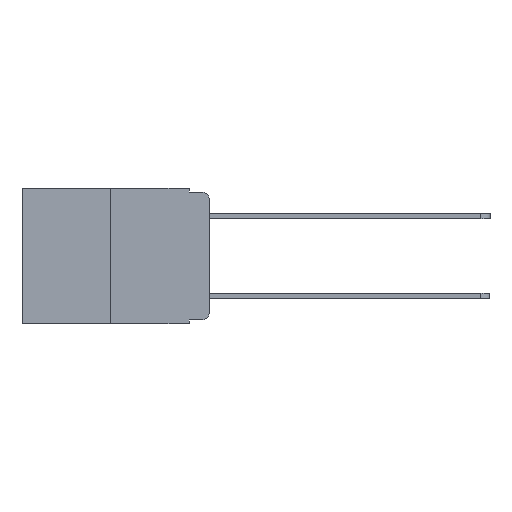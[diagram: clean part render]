
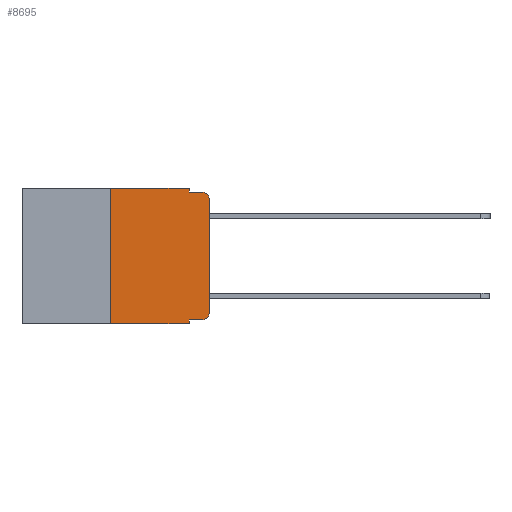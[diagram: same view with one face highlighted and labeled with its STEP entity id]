
A CAD part, left-side view. The second image highlights one B-rep face of the part: STEP entity #8695.
In plain terms, the highlighted planar face has unit normal (-1, 0, 0).
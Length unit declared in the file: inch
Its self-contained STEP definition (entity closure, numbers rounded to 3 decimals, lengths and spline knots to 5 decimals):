
#64 = LINE ( 'NONE', #6780, #10073 ) ;
#227 = EDGE_LOOP ( 'NONE', ( #10175, #6508, #6427, #11530, #5528, #4288, #5769, #5811, #8280, #3083 ) ) ;
#382 = VERTEX_POINT ( 'NONE', #4713 ) ;
#872 = VECTOR ( 'NONE', #7468, 39.37008 ) ;
#919 = CARTESIAN_POINT ( 'NONE',  ( 0., 0.051, 0. ) ) ;
#1020 = VERTEX_POINT ( 'NONE', #5211 ) ;
#1078 = VECTOR ( 'NONE', #2235, 39.37008 ) ;
#1082 = DIRECTION ( 'NONE',  ( 0., 0., 1. ) ) ;
#1133 = DIRECTION ( 'NONE',  ( 1., 0., 0. ) ) ;
#1198 = LINE ( 'NONE', #2793, #872 ) ;
#1311 = VERTEX_POINT ( 'NONE', #11874 ) ;
#1680 = AXIS2_PLACEMENT_3D ( 'NONE', #5020, #1133, #7869 ) ;
#1863 = EDGE_CURVE ( 'NONE', #1311, #4273, #8727, .T. ) ;
#1935 = CARTESIAN_POINT ( 'NONE',  ( 0., 0.473, 0. ) ) ;
#2045 = CARTESIAN_POINT ( 'NONE',  ( 0., 0.25, 0. ) ) ;
#2103 = VERTEX_POINT ( 'NONE', #4252 ) ;
#2163 = CIRCLE ( 'NONE', #2582, 0.02 ) ;
#2187 = CARTESIAN_POINT ( 'NONE',  ( 0., 0.02, -0.333 ) ) ;
#2235 = DIRECTION ( 'NONE',  ( 0., -1., 0. ) ) ;
#2582 = AXIS2_PLACEMENT_3D ( 'NONE', #10683, #5071, #11583 ) ;
#2793 = CARTESIAN_POINT ( 'NONE',  ( 0., 0.051, 0. ) ) ;
#2950 = VECTOR ( 'NONE', #11321, 39.37008 ) ;
#3000 = DIRECTION ( 'NONE',  ( 0., 0., 1. ) ) ;
#3038 = CARTESIAN_POINT ( 'NONE',  ( 0., 0.051, -0.343 ) ) ;
#3083 = ORIENTED_EDGE ( 'NONE', *, *, #5083, .T. ) ;
#3202 = VERTEX_POINT ( 'NONE', #2187 ) ;
#3207 = EDGE_CURVE ( 'NONE', #2103, #9850, #8780, .T. ) ;
#3277 = DIRECTION ( 'NONE',  ( -1., 0., 0. ) ) ;
#3634 = EDGE_CURVE ( 'NONE', #382, #4273, #64, .T. ) ;
#3652 = VERTEX_POINT ( 'NONE', #2045 ) ;
#3711 = CARTESIAN_POINT ( 'NONE',  ( 0., 0.051, -0.333 ) ) ;
#3979 = DIRECTION ( 'NONE',  ( 0., 0., -1. ) ) ;
#4140 = LINE ( 'NONE', #11490, #10984 ) ;
#4190 = FACE_OUTER_BOUND ( 'NONE', #227, .T. ) ;
#4252 = CARTESIAN_POINT ( 'NONE',  ( 0., 0.25, -0.343 ) ) ;
#4273 = VERTEX_POINT ( 'NONE', #6560 ) ;
#4288 = ORIENTED_EDGE ( 'NONE', *, *, #11700, .F. ) ;
#4647 = DIRECTION ( 'NONE',  ( 0., -1., 0. ) ) ;
#4713 = CARTESIAN_POINT ( 'NONE',  ( 0., 0.051, -0.01 ) ) ;
#4741 = EDGE_CURVE ( 'NONE', #1020, #382, #1198, .T. ) ;
#5020 = CARTESIAN_POINT ( 'NONE',  ( 0., 0.473, 0. ) ) ;
#5071 = DIRECTION ( 'NONE',  ( -1., 0., 0. ) ) ;
#5083 = EDGE_CURVE ( 'NONE', #3202, #6679, #2163, .T. ) ;
#5211 = CARTESIAN_POINT ( 'NONE',  ( 0., 0.051, 0. ) ) ;
#5463 = VERTEX_POINT ( 'NONE', #3711 ) ;
#5528 = ORIENTED_EDGE ( 'NONE', *, *, #11068, .F. ) ;
#5769 = ORIENTED_EDGE ( 'NONE', *, *, #3207, .T. ) ;
#5811 = ORIENTED_EDGE ( 'NONE', *, *, #7048, .F. ) ;
#6030 = LINE ( 'NONE', #1935, #2950 ) ;
#6427 = ORIENTED_EDGE ( 'NONE', *, *, #3634, .F. ) ;
#6508 = ORIENTED_EDGE ( 'NONE', *, *, #1863, .T. ) ;
#6560 = CARTESIAN_POINT ( 'NONE',  ( 0., 0.02, -0.01 ) ) ;
#6679 = VERTEX_POINT ( 'NONE', #11732 ) ;
#6780 = CARTESIAN_POINT ( 'NONE',  ( 0., 0.051, -0.01 ) ) ;
#6912 = PLANE ( 'NONE',  #1680 ) ;
#6954 = CARTESIAN_POINT ( 'NONE',  ( 0., 0.473, -0.343 ) ) ;
#7048 = EDGE_CURVE ( 'NONE', #5463, #9850, #10271, .T. ) ;
#7468 = DIRECTION ( 'NONE',  ( 0., 0., -1. ) ) ;
#7778 = VECTOR ( 'NONE', #10492, 39.37008 ) ;
#7869 = DIRECTION ( 'NONE',  ( 0., 0., -1. ) ) ;
#8280 = ORIENTED_EDGE ( 'NONE', *, *, #12105, .T. ) ;
#8682 = VECTOR ( 'NONE', #4647, 39.37008 ) ;
#8695 = ADVANCED_FACE ( 'NONE', ( #4190 ), #6912, .F. ) ;
#8718 = DIRECTION ( 'NONE',  ( 0., -1., 0. ) ) ;
#8727 = CIRCLE ( 'NONE', #10660, 0.02 ) ;
#8780 = LINE ( 'NONE', #6954, #1078 ) ;
#9369 = CARTESIAN_POINT ( 'NONE',  ( 0., 0.051, -0.333 ) ) ;
#9582 = CARTESIAN_POINT ( 'NONE',  ( 0., 0.25, 0. ) ) ;
#9718 = CARTESIAN_POINT ( 'NONE',  ( 0., 0.02, -0.03 ) ) ;
#9850 = VERTEX_POINT ( 'NONE', #3038 ) ;
#10000 = VECTOR ( 'NONE', #3000, 39.37008 ) ;
#10073 = VECTOR ( 'NONE', #8718, 39.37008 ) ;
#10175 = ORIENTED_EDGE ( 'NONE', *, *, #10593, .T. ) ;
#10271 = LINE ( 'NONE', #919, #7778 ) ;
#10492 = DIRECTION ( 'NONE',  ( 0., 0., -1. ) ) ;
#10593 = EDGE_CURVE ( 'NONE', #6679, #1311, #4140, .T. ) ;
#10660 = AXIS2_PLACEMENT_3D ( 'NONE', #9718, #3277, #3979 ) ;
#10683 = CARTESIAN_POINT ( 'NONE',  ( 0., 0.02, -0.313 ) ) ;
#10984 = VECTOR ( 'NONE', #1082, 39.37008 ) ;
#11068 = EDGE_CURVE ( 'NONE', #3652, #1020, #6030, .T. ) ;
#11086 = LINE ( 'NONE', #9369, #8682 ) ;
#11321 = DIRECTION ( 'NONE',  ( 0., -1., 0. ) ) ;
#11490 = CARTESIAN_POINT ( 'NONE',  ( 0., 0., 0. ) ) ;
#11530 = ORIENTED_EDGE ( 'NONE', *, *, #4741, .F. ) ;
#11583 = DIRECTION ( 'NONE',  ( 0., 0., -1. ) ) ;
#11700 = EDGE_CURVE ( 'NONE', #2103, #3652, #12308, .T. ) ;
#11732 = CARTESIAN_POINT ( 'NONE',  ( 0., 0., -0.313 ) ) ;
#11874 = CARTESIAN_POINT ( 'NONE',  ( 0., 0., -0.03 ) ) ;
#12105 = EDGE_CURVE ( 'NONE', #5463, #3202, #11086, .T. ) ;
#12308 = LINE ( 'NONE', #9582, #10000 ) ;
